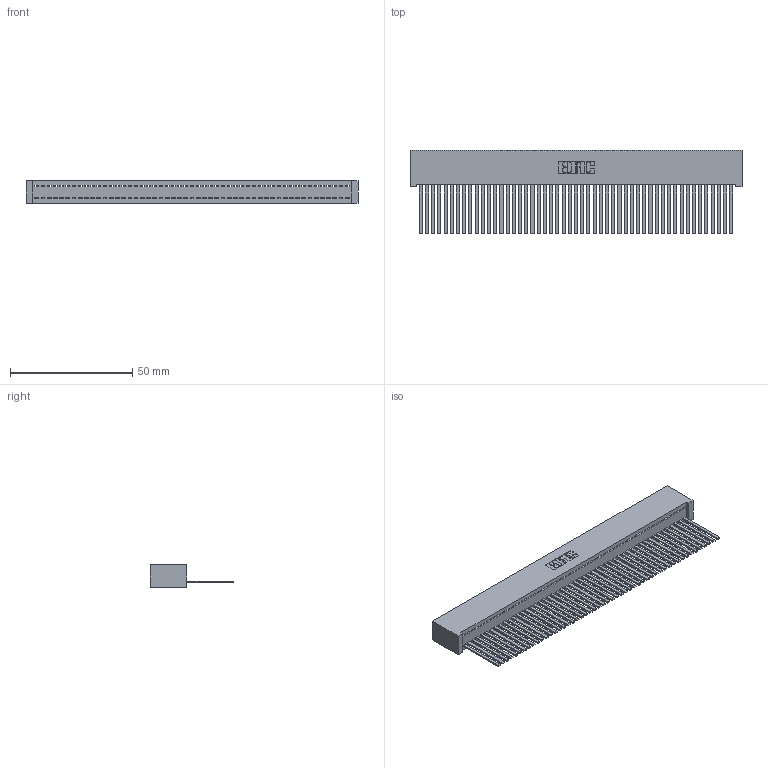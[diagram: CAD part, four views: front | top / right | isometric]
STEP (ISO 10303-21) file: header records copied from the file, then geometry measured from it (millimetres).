
FILE_DESCRIPTION (( 'STEP AP203' ), '1' );
FILE_NAME ('342-051-544-101.STEP', '2019-10-03T00:37:42', ( '' ), ( '' ), 'SwSTEP 2.0', 'SolidWorks 2016', '' );
FILE_SCHEMA (( 'CONFIG_CONTROL_DESIGN' ));
Length unit declared in the file: inch
Products named in the file (3): 342 Part_Lugless; 345-292-001_345-293-144; 342-051-544-101
Assembly tree (52 placements, depth 2):
  342-051-544-101
    342 Part_Lugless
    345-292-001_345-293-144  x51
Bounding box: 135.79 x 34.3 x 9.4 mm (x, y, z)
Volume: 12938.7 mm3; surface area: 21172.3 mm2
Topology: 52 solids, 52 shells, 2754 faces, 8333 edges, 5486 vertices
Faces by surface type: plane 2000, cylinder 754
Entity records: 29421 total; most frequent: CARTESIAN_POINT 5079, ORIENTED_EDGE 5066, DIRECTION 4255, EDGE_CURVE 2533, VECTOR 2417, LINE 2417, VERTEX_POINT 1686, AXIS2_PLACEMENT_3D 919
